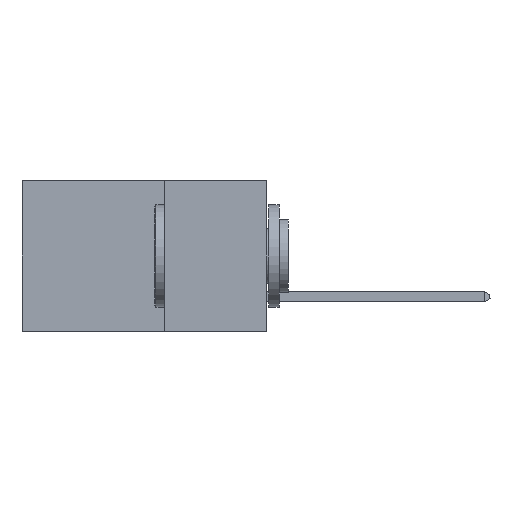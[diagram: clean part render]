
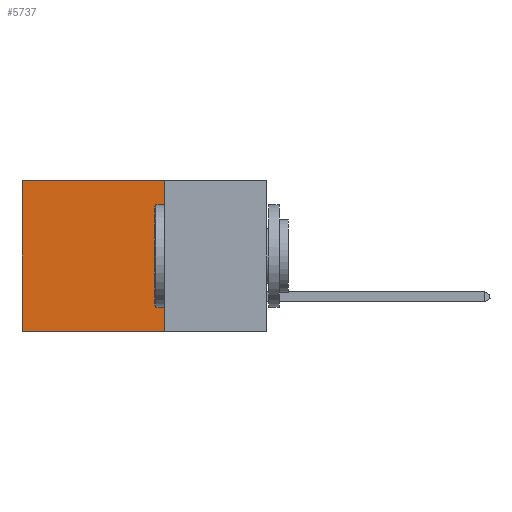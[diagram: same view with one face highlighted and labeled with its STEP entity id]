
A CAD part, left-side view. The second image highlights one B-rep face of the part: STEP entity #5737.
In plain terms, the highlighted planar face has unit normal (-1, 0, 0).
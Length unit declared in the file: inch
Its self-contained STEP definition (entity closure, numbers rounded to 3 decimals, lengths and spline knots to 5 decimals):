
#8 = LINE ( 'NONE', #7316, #455 ) ;
#455 = VECTOR ( 'NONE', #7258, 39.37008 ) ;
#1028 = EDGE_CURVE ( 'NONE', #4328, #6421, #2523, .T. ) ;
#1206 = CARTESIAN_POINT ( 'NONE',  ( 0.2875, 0.6, 0. ) ) ;
#2515 = VERTEX_POINT ( 'NONE', #1206 ) ;
#2523 = LINE ( 'NONE', #14210, #16395 ) ;
#2665 = EDGE_LOOP ( 'NONE', ( #15880, #15981, #15501, #8517 ) ) ;
#3106 = EDGE_CURVE ( 'NONE', #8972, #2515, #8, .T. ) ;
#3281 = CARTESIAN_POINT ( 'NONE',  ( 0.2875, 0.25, 0. ) ) ;
#3804 = DIRECTION ( 'NONE',  ( 0., 0., -1. ) ) ;
#4159 = LINE ( 'NONE', #7431, #7740 ) ;
#4328 = VERTEX_POINT ( 'NONE', #15712 ) ;
#5737 = ADVANCED_FACE ( 'NONE', ( #14204 ), #14511, .F. ) ;
#6321 = VECTOR ( 'NONE', #10010, 39.37008 ) ;
#6421 = VERTEX_POINT ( 'NONE', #14916 ) ;
#7258 = DIRECTION ( 'NONE',  ( 0., 1., 0. ) ) ;
#7316 = CARTESIAN_POINT ( 'NONE',  ( 0.2875, 0.25, 0. ) ) ;
#7431 = CARTESIAN_POINT ( 'NONE',  ( 0.2875, 0.6, 0. ) ) ;
#7740 = VECTOR ( 'NONE', #16735, 39.37008 ) ;
#8361 = EDGE_CURVE ( 'NONE', #8972, #4328, #10325, .T. ) ;
#8517 = ORIENTED_EDGE ( 'NONE', *, *, #3106, .T. ) ;
#8581 = CARTESIAN_POINT ( 'NONE',  ( 0.2875, 0.25, 0. ) ) ;
#8972 = VERTEX_POINT ( 'NONE', #8581 ) ;
#9172 = CARTESIAN_POINT ( 'NONE',  ( 0.2875, 0.25, 0. ) ) ;
#9783 = EDGE_CURVE ( 'NONE', #2515, #6421, #4159, .T. ) ;
#10010 = DIRECTION ( 'NONE',  ( 0., 0., -1. ) ) ;
#10325 = LINE ( 'NONE', #3281, #6321 ) ;
#11870 = DIRECTION ( 'NONE',  ( 1., 0., 0. ) ) ;
#12923 = DIRECTION ( 'NONE',  ( 0., 1., 0. ) ) ;
#14204 = FACE_OUTER_BOUND ( 'NONE', #2665, .T. ) ;
#14210 = CARTESIAN_POINT ( 'NONE',  ( 0.2875, 0.25, -0.37 ) ) ;
#14511 = PLANE ( 'NONE',  #15839 ) ;
#14916 = CARTESIAN_POINT ( 'NONE',  ( 0.2875, 0.6, -0.37 ) ) ;
#15501 = ORIENTED_EDGE ( 'NONE', *, *, #8361, .F. ) ;
#15712 = CARTESIAN_POINT ( 'NONE',  ( 0.2875, 0.25, -0.37 ) ) ;
#15839 = AXIS2_PLACEMENT_3D ( 'NONE', #9172, #11870, #3804 ) ;
#15880 = ORIENTED_EDGE ( 'NONE', *, *, #9783, .T. ) ;
#15981 = ORIENTED_EDGE ( 'NONE', *, *, #1028, .F. ) ;
#16395 = VECTOR ( 'NONE', #12923, 39.37008 ) ;
#16735 = DIRECTION ( 'NONE',  ( 0., 0., -1. ) ) ;
